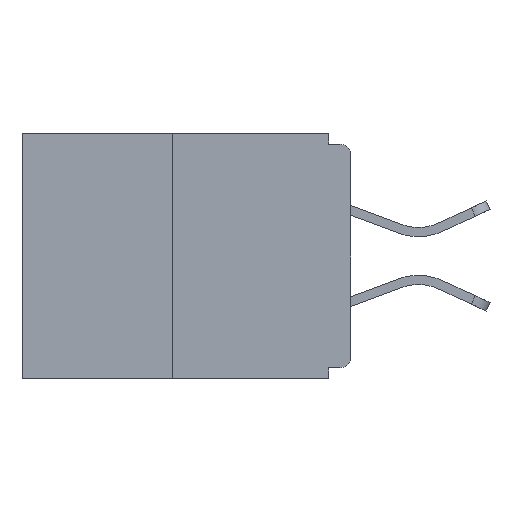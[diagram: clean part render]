
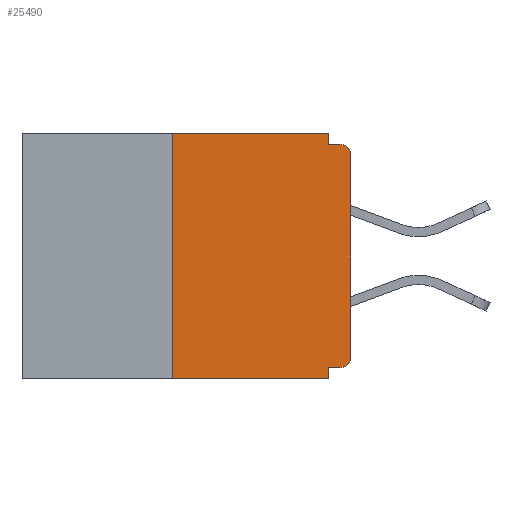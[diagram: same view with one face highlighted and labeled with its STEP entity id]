
A CAD part, left-side view. The second image highlights one B-rep face of the part: STEP entity #25490.
In plain terms, the highlighted planar face has unit normal (-1, 0, 0).
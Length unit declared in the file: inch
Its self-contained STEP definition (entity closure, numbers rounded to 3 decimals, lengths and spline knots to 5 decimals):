
#580 = ORIENTED_EDGE ( 'NONE', *, *, #22330, .T. ) ;
#614 = EDGE_CURVE ( 'NONE', #17568, #26900, #12044, .T. ) ;
#699 = AXIS2_PLACEMENT_3D ( 'NONE', #2030, #6325, #8548 ) ;
#1181 = CARTESIAN_POINT ( 'NONE',  ( 0., 0.25, 0. ) ) ;
#1330 = VERTEX_POINT ( 'NONE', #9878 ) ;
#1436 = LINE ( 'NONE', #20265, #20262 ) ;
#1953 = LINE ( 'NONE', #20342, #17706 ) ;
#2006 = ORIENTED_EDGE ( 'NONE', *, *, #12123, .T. ) ;
#2030 = CARTESIAN_POINT ( 'NONE',  ( 0., 0.46, 0. ) ) ;
#2393 = DIRECTION ( 'NONE',  ( 0., -1., 0. ) ) ;
#2793 = VECTOR ( 'NONE', #13888, 39.37008 ) ;
#2851 = LINE ( 'NONE', #14919, #21030 ) ;
#3402 = CARTESIAN_POINT ( 'NONE',  ( 0., 0.25, -0.343 ) ) ;
#3817 = EDGE_CURVE ( 'NONE', #17568, #27888, #20031, .T. ) ;
#4337 = VERTEX_POINT ( 'NONE', #17851 ) ;
#5092 = DIRECTION ( 'NONE',  ( -1., 0., 0. ) ) ;
#5570 = EDGE_CURVE ( 'NONE', #21687, #6674, #10235, .T. ) ;
#5873 = AXIS2_PLACEMENT_3D ( 'NONE', #26765, #5092, #22675 ) ;
#6325 = DIRECTION ( 'NONE',  ( 1., 0., 0. ) ) ;
#6585 = CARTESIAN_POINT ( 'NONE',  ( 0., 0., -0.015 ) ) ;
#6674 = VERTEX_POINT ( 'NONE', #12445 ) ;
#6701 = CARTESIAN_POINT ( 'NONE',  ( 0., 0.46, 0. ) ) ;
#8183 = CARTESIAN_POINT ( 'NONE',  ( 0., 0.031, -0.343 ) ) ;
#8272 = LINE ( 'NONE', #6701, #9272 ) ;
#8548 = DIRECTION ( 'NONE',  ( 0., 0., -1. ) ) ;
#9050 = CARTESIAN_POINT ( 'NONE',  ( 0., 0.031, -0.015 ) ) ;
#9272 = VECTOR ( 'NONE', #13424, 39.37008 ) ;
#9878 = CARTESIAN_POINT ( 'NONE',  ( 0., 0.031, 0. ) ) ;
#10235 = LINE ( 'NONE', #6585, #20862 ) ;
#10660 = ORIENTED_EDGE ( 'NONE', *, *, #11912, .F. ) ;
#11912 = EDGE_CURVE ( 'NONE', #1330, #21687, #18885, .T. ) ;
#11997 = ORIENTED_EDGE ( 'NONE', *, *, #614, .T. ) ;
#12035 = CARTESIAN_POINT ( 'NONE',  ( 0., 0., -0.03 ) ) ;
#12044 = LINE ( 'NONE', #20285, #2793 ) ;
#12123 = EDGE_CURVE ( 'NONE', #12670, #6674, #24352, .T. ) ;
#12445 = CARTESIAN_POINT ( 'NONE',  ( 0., 0.015, -0.015 ) ) ;
#12555 = VERTEX_POINT ( 'NONE', #15780 ) ;
#12670 = VERTEX_POINT ( 'NONE', #12035 ) ;
#12909 = ORIENTED_EDGE ( 'NONE', *, *, #23642, .F. ) ;
#13076 = VERTEX_POINT ( 'NONE', #17228 ) ;
#13290 = EDGE_LOOP ( 'NONE', ( #12909, #15548, #11997, #20874, #16765, #21145, #580, #2006, #15823, #10660 ) ) ;
#13424 = DIRECTION ( 'NONE',  ( 0., -1., 0. ) ) ;
#13566 = DIRECTION ( 'NONE',  ( 0., 0., -1. ) ) ;
#13888 = DIRECTION ( 'NONE',  ( 0., -1., 0. ) ) ;
#14434 = DIRECTION ( 'NONE',  ( -1., 0., 0. ) ) ;
#14768 = EDGE_CURVE ( 'NONE', #12555, #4337, #1953, .T. ) ;
#14919 = CARTESIAN_POINT ( 'NONE',  ( 0., 0., 0. ) ) ;
#15126 = VECTOR ( 'NONE', #13566, 39.37008 ) ;
#15548 = ORIENTED_EDGE ( 'NONE', *, *, #3817, .F. ) ;
#15780 = CARTESIAN_POINT ( 'NONE',  ( 0., 0.015, -0.328 ) ) ;
#15823 = ORIENTED_EDGE ( 'NONE', *, *, #5570, .F. ) ;
#16061 = DIRECTION ( 'NONE',  ( 0., 1., 0. ) ) ;
#16562 = DIRECTION ( 'NONE',  ( 0., 0., -1. ) ) ;
#16765 = ORIENTED_EDGE ( 'NONE', *, *, #14768, .F. ) ;
#16982 = EDGE_CURVE ( 'NONE', #12555, #13076, #25772, .T. ) ;
#17228 = CARTESIAN_POINT ( 'NONE',  ( 0., 0., -0.313 ) ) ;
#17568 = VERTEX_POINT ( 'NONE', #3402 ) ;
#17667 = VECTOR ( 'NONE', #27531, 39.37008 ) ;
#17706 = VECTOR ( 'NONE', #16061, 39.37008 ) ;
#17851 = CARTESIAN_POINT ( 'NONE',  ( 0., 0.031, -0.328 ) ) ;
#18885 = LINE ( 'NONE', #24199, #15126 ) ;
#20031 = LINE ( 'NONE', #1181, #17667 ) ;
#20262 = VECTOR ( 'NONE', #26518, 39.37008 ) ;
#20265 = CARTESIAN_POINT ( 'NONE',  ( 0., 0.031, -0.343 ) ) ;
#20285 = CARTESIAN_POINT ( 'NONE',  ( 0., 0.46, -0.343 ) ) ;
#20342 = CARTESIAN_POINT ( 'NONE',  ( 0., 0., -0.328 ) ) ;
#20358 = FACE_OUTER_BOUND ( 'NONE', #13290, .T. ) ;
#20862 = VECTOR ( 'NONE', #2393, 39.37008 ) ;
#20874 = ORIENTED_EDGE ( 'NONE', *, *, #23048, .F. ) ;
#21030 = VECTOR ( 'NONE', #27664, 39.37008 ) ;
#21145 = ORIENTED_EDGE ( 'NONE', *, *, #16982, .T. ) ;
#21440 = AXIS2_PLACEMENT_3D ( 'NONE', #22959, #14434, #16562 ) ;
#21687 = VERTEX_POINT ( 'NONE', #9050 ) ;
#22330 = EDGE_CURVE ( 'NONE', #13076, #12670, #2851, .T. ) ;
#22675 = DIRECTION ( 'NONE',  ( 0., 0., -1. ) ) ;
#22959 = CARTESIAN_POINT ( 'NONE',  ( 0., 0.015, -0.313 ) ) ;
#23048 = EDGE_CURVE ( 'NONE', #4337, #26900, #1436, .T. ) ;
#23642 = EDGE_CURVE ( 'NONE', #27888, #1330, #8272, .T. ) ;
#24199 = CARTESIAN_POINT ( 'NONE',  ( 0., 0.031, 0. ) ) ;
#24352 = CIRCLE ( 'NONE', #5873, 0.015 ) ;
#25490 = ADVANCED_FACE ( 'NONE', ( #20358 ), #25768, .F. ) ;
#25768 = PLANE ( 'NONE',  #699 ) ;
#25772 = CIRCLE ( 'NONE', #21440, 0.015 ) ;
#26518 = DIRECTION ( 'NONE',  ( 0., 0., -1. ) ) ;
#26765 = CARTESIAN_POINT ( 'NONE',  ( 0., 0.015, -0.03 ) ) ;
#26900 = VERTEX_POINT ( 'NONE', #8183 ) ;
#27487 = CARTESIAN_POINT ( 'NONE',  ( 0., 0.25, 0. ) ) ;
#27531 = DIRECTION ( 'NONE',  ( 0., 0., 1. ) ) ;
#27664 = DIRECTION ( 'NONE',  ( 0., 0., 1. ) ) ;
#27888 = VERTEX_POINT ( 'NONE', #27487 ) ;
